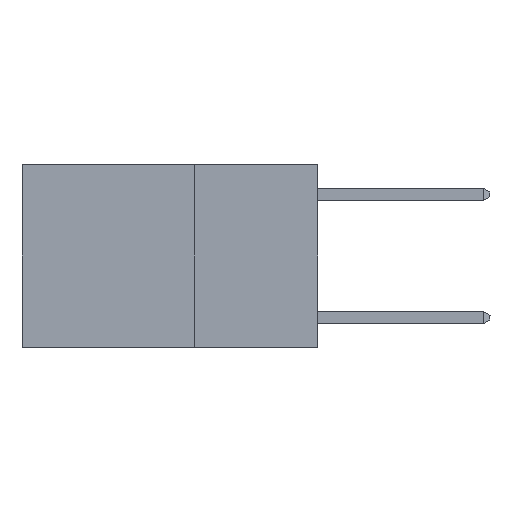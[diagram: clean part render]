
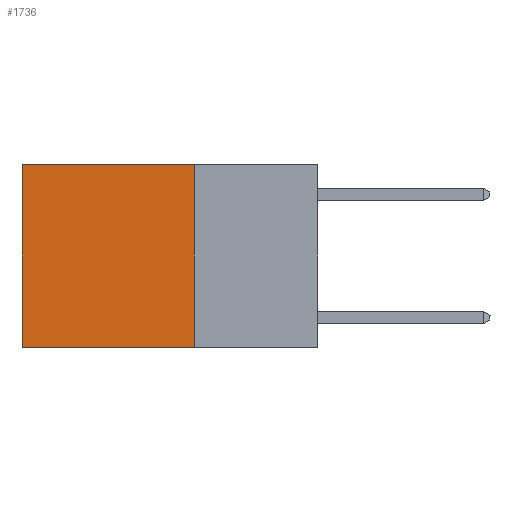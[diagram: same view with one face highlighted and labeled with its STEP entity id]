
A CAD part, left-side view. The second image highlights one B-rep face of the part: STEP entity #1736.
In plain terms, the highlighted planar face has unit normal (-1, 0, 0).
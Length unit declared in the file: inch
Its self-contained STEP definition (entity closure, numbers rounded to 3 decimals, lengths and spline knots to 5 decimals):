
#235 = CARTESIAN_POINT ( 'NONE',  ( 0.2625, 0.25, 0. ) ) ;
#935 = LINE ( 'NONE', #15797, #1906 ) ;
#1239 = EDGE_CURVE ( 'NONE', #17338, #2847, #935, .T. ) ;
#1307 = ORIENTED_EDGE ( 'NONE', *, *, #10143, .T. ) ;
#1491 = ORIENTED_EDGE ( 'NONE', *, *, #14303, .F. ) ;
#1736 = ADVANCED_FACE ( 'NONE', ( #10273 ), #14242, .F. ) ;
#1906 = VECTOR ( 'NONE', #10414, 39.37008 ) ;
#2117 = CARTESIAN_POINT ( 'NONE',  ( 0.2625, 0.25, 0. ) ) ;
#2409 = LINE ( 'NONE', #7432, #17389 ) ;
#2847 = VERTEX_POINT ( 'NONE', #7166 ) ;
#2937 = VERTEX_POINT ( 'NONE', #11797 ) ;
#3574 = DIRECTION ( 'NONE',  ( 0., 0., -1. ) ) ;
#3702 = VERTEX_POINT ( 'NONE', #14850 ) ;
#4618 = ORIENTED_EDGE ( 'NONE', *, *, #12087, .F. ) ;
#6208 = CARTESIAN_POINT ( 'NONE',  ( 0.2625, 0.6, 0. ) ) ;
#6426 = DIRECTION ( 'NONE',  ( 0., 0., -1. ) ) ;
#7166 = CARTESIAN_POINT ( 'NONE',  ( 0.2625, 0.6, 0. ) ) ;
#7432 = CARTESIAN_POINT ( 'NONE',  ( 0.2625, 0.25, -0.37 ) ) ;
#8681 = VECTOR ( 'NONE', #3574, 39.37008 ) ;
#8791 = VECTOR ( 'NONE', #14305, 39.37008 ) ;
#8821 = LINE ( 'NONE', #6208, #8681 ) ;
#8826 = DIRECTION ( 'NONE',  ( 0., 1., 0. ) ) ;
#10143 = EDGE_CURVE ( 'NONE', #2847, #3702, #8821, .T. ) ;
#10273 = FACE_OUTER_BOUND ( 'NONE', #14150, .T. ) ;
#10414 = DIRECTION ( 'NONE',  ( 0., 1., 0. ) ) ;
#11206 = CARTESIAN_POINT ( 'NONE',  ( 0.2625, 0.25, 0. ) ) ;
#11797 = CARTESIAN_POINT ( 'NONE',  ( 0.2625, 0.25, -0.37 ) ) ;
#12087 = EDGE_CURVE ( 'NONE', #2937, #3702, #2409, .T. ) ;
#13714 = ORIENTED_EDGE ( 'NONE', *, *, #1239, .T. ) ;
#14150 = EDGE_LOOP ( 'NONE', ( #1307, #4618, #1491, #13714 ) ) ;
#14242 = PLANE ( 'NONE',  #16637 ) ;
#14303 = EDGE_CURVE ( 'NONE', #17338, #2937, #15013, .T. ) ;
#14305 = DIRECTION ( 'NONE',  ( 0., 0., -1. ) ) ;
#14850 = CARTESIAN_POINT ( 'NONE',  ( 0.2625, 0.6, -0.37 ) ) ;
#15013 = LINE ( 'NONE', #235, #8791 ) ;
#15767 = DIRECTION ( 'NONE',  ( 1., 0., 0. ) ) ;
#15797 = CARTESIAN_POINT ( 'NONE',  ( 0.2625, 0.25, 0. ) ) ;
#16637 = AXIS2_PLACEMENT_3D ( 'NONE', #2117, #15767, #6426 ) ;
#17338 = VERTEX_POINT ( 'NONE', #11206 ) ;
#17389 = VECTOR ( 'NONE', #8826, 39.37008 ) ;
